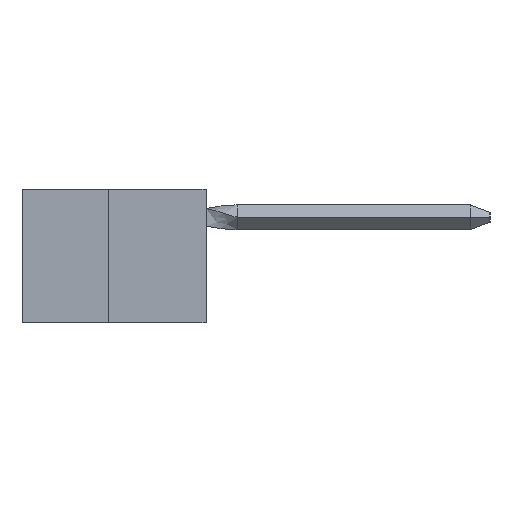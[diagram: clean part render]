
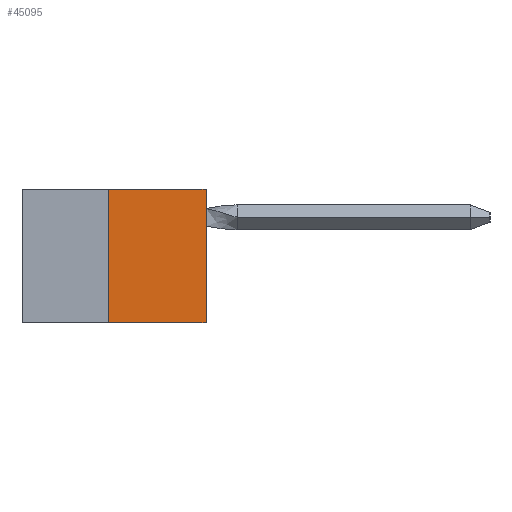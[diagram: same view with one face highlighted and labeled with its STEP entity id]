
A CAD part, left-side view. The second image highlights one B-rep face of the part: STEP entity #45095.
In plain terms, the highlighted planar face has unit normal (-1, 0, 0).
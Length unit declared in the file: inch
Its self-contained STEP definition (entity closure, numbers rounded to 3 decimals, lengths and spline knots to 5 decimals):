
#190 = EDGE_CURVE ( 'NONE', #20918, #35575, #24169, .T. ) ;
#928 = EDGE_CURVE ( 'NONE', #35575, #9622, #6889, .T. ) ;
#4728 = CARTESIAN_POINT ( 'NONE',  ( 0., 0., -0.343 ) ) ;
#6889 = LINE ( 'NONE', #55093, #29515 ) ;
#8171 = ORIENTED_EDGE ( 'NONE', *, *, #46190, .T. ) ;
#9618 = VECTOR ( 'NONE', #16128, 39.37008 ) ;
#9622 = VERTEX_POINT ( 'NONE', #31103 ) ;
#10452 = CARTESIAN_POINT ( 'NONE',  ( 0., 0., 0. ) ) ;
#10966 = CARTESIAN_POINT ( 'NONE',  ( 0., 0.473, -0.343 ) ) ;
#11186 = FACE_OUTER_BOUND ( 'NONE', #13809, .T. ) ;
#12220 = LINE ( 'NONE', #10966, #49453 ) ;
#12349 = VERTEX_POINT ( 'NONE', #4728 ) ;
#13809 = EDGE_LOOP ( 'NONE', ( #52017, #27725, #34917, #8171 ) ) ;
#14490 = DIRECTION ( 'NONE',  ( 0., -1., 0. ) ) ;
#16128 = DIRECTION ( 'NONE',  ( 0., 0., 1. ) ) ;
#19457 = PLANE ( 'NONE',  #49684 ) ;
#20918 = VERTEX_POINT ( 'NONE', #27075 ) ;
#23932 = DIRECTION ( 'NONE',  ( 1., 0., 0. ) ) ;
#24132 = CARTESIAN_POINT ( 'NONE',  ( 0., 0.25, 0. ) ) ;
#24169 = LINE ( 'NONE', #24132, #9618 ) ;
#27075 = CARTESIAN_POINT ( 'NONE',  ( 0., 0.25, -0.343 ) ) ;
#27725 = ORIENTED_EDGE ( 'NONE', *, *, #190, .F. ) ;
#29515 = VECTOR ( 'NONE', #46379, 39.37008 ) ;
#29754 = EDGE_CURVE ( 'NONE', #20918, #12349, #12220, .T. ) ;
#30814 = CARTESIAN_POINT ( 'NONE',  ( 0., 0.25, 0. ) ) ;
#31103 = CARTESIAN_POINT ( 'NONE',  ( 0., 0., 0. ) ) ;
#31871 = CARTESIAN_POINT ( 'NONE',  ( 0., 0.473, 0. ) ) ;
#31943 = DIRECTION ( 'NONE',  ( 0., 0., 1. ) ) ;
#32254 = VECTOR ( 'NONE', #31943, 39.37008 ) ;
#32608 = DIRECTION ( 'NONE',  ( 0., 0., -1. ) ) ;
#34917 = ORIENTED_EDGE ( 'NONE', *, *, #29754, .T. ) ;
#35575 = VERTEX_POINT ( 'NONE', #30814 ) ;
#44246 = LINE ( 'NONE', #10452, #32254 ) ;
#45095 = ADVANCED_FACE ( 'NONE', ( #11186 ), #19457, .F. ) ;
#46190 = EDGE_CURVE ( 'NONE', #12349, #9622, #44246, .T. ) ;
#46379 = DIRECTION ( 'NONE',  ( 0., -1., 0. ) ) ;
#49453 = VECTOR ( 'NONE', #14490, 39.37008 ) ;
#49684 = AXIS2_PLACEMENT_3D ( 'NONE', #31871, #23932, #32608 ) ;
#52017 = ORIENTED_EDGE ( 'NONE', *, *, #928, .F. ) ;
#55093 = CARTESIAN_POINT ( 'NONE',  ( 0., 0.473, 0. ) ) ;
